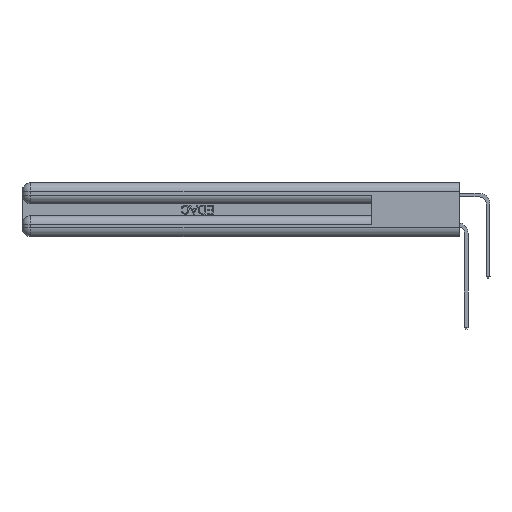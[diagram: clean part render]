
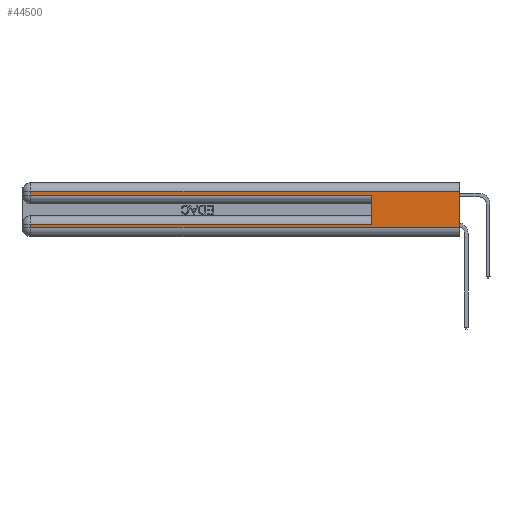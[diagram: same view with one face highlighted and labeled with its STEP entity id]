
A CAD part, left-side view. The second image highlights one B-rep face of the part: STEP entity #44500.
In plain terms, the highlighted planar face has unit normal (-1, 0, 0).
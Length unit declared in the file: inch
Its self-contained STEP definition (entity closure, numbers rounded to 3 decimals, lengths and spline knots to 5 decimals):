
#32 = LINE ( 'NONE', #15522, #5811 ) ;
#639 = VECTOR ( 'NONE', #29150, 39.37008 ) ;
#672 = VECTOR ( 'NONE', #7883, 39.37008 ) ;
#2820 = EDGE_CURVE ( 'NONE', #15118, #32113, #42687, .T. ) ;
#3298 = VERTEX_POINT ( 'NONE', #42536 ) ;
#4163 = VERTEX_POINT ( 'NONE', #35458 ) ;
#4342 = CARTESIAN_POINT ( 'NONE',  ( 0., 0., 0.31 ) ) ;
#5330 = DIRECTION ( 'NONE',  ( 0., 0., -1. ) ) ;
#5811 = VECTOR ( 'NONE', #40610, 39.37008 ) ;
#5870 = CARTESIAN_POINT ( 'NONE',  ( 0., 0., 0.06 ) ) ;
#6993 = AXIS2_PLACEMENT_3D ( 'NONE', #20928, #46917, #7192 ) ;
#7192 = DIRECTION ( 'NONE',  ( 0., 0., -1. ) ) ;
#7569 = LINE ( 'NONE', #17397, #22029 ) ;
#7586 = DIRECTION ( 'NONE',  ( 0., 0., -1. ) ) ;
#7883 = DIRECTION ( 'NONE',  ( 0., 1., 0. ) ) ;
#8576 = ORIENTED_EDGE ( 'NONE', *, *, #2820, .T. ) ;
#9760 = ORIENTED_EDGE ( 'NONE', *, *, #25364, .T. ) ;
#10143 = LINE ( 'NONE', #27771, #14815 ) ;
#13827 = DIRECTION ( 'NONE',  ( 0., 1., 0. ) ) ;
#13920 = LINE ( 'NONE', #4342, #672 ) ;
#14439 = VECTOR ( 'NONE', #7586, 39.37008 ) ;
#14815 = VECTOR ( 'NONE', #5330, 39.37008 ) ;
#15118 = VERTEX_POINT ( 'NONE', #22848 ) ;
#15131 = VERTEX_POINT ( 'NONE', #5870 ) ;
#15522 = CARTESIAN_POINT ( 'NONE',  ( 0., 2.94, 0.37 ) ) ;
#17222 = EDGE_CURVE ( 'NONE', #34478, #18500, #39340, .T. ) ;
#17397 = CARTESIAN_POINT ( 'NONE',  ( 0., 0., 0.085 ) ) ;
#18054 = EDGE_CURVE ( 'NONE', #20332, #4163, #32, .T. ) ;
#18500 = VERTEX_POINT ( 'NONE', #32402 ) ;
#20332 = VERTEX_POINT ( 'NONE', #34248 ) ;
#20928 = CARTESIAN_POINT ( 'NONE',  ( 0., 0., 0.37 ) ) ;
#21116 = EDGE_CURVE ( 'NONE', #3298, #15131, #10143, .T. ) ;
#21173 = ORIENTED_EDGE ( 'NONE', *, *, #21116, .F. ) ;
#21985 = CARTESIAN_POINT ( 'NONE',  ( 0., 0.6, 0.085 ) ) ;
#22029 = VECTOR ( 'NONE', #13827, 39.37008 ) ;
#22497 = EDGE_LOOP ( 'NONE', ( #21173, #37369, #8576, #9760, #22871, #39347, #37318, #46842 ) ) ;
#22683 = CARTESIAN_POINT ( 'NONE',  ( 0., 2.94, 0.37 ) ) ;
#22848 = CARTESIAN_POINT ( 'NONE',  ( 0., 2.94, 0.31 ) ) ;
#22871 = ORIENTED_EDGE ( 'NONE', *, *, #17222, .F. ) ;
#23947 = EDGE_CURVE ( 'NONE', #34478, #20332, #7569, .T. ) ;
#24166 = FACE_OUTER_BOUND ( 'NONE', #22497, .T. ) ;
#25364 = EDGE_CURVE ( 'NONE', #32113, #18500, #36343, .T. ) ;
#27719 = CARTESIAN_POINT ( 'NONE',  ( 0., 0., 0.06 ) ) ;
#27771 = CARTESIAN_POINT ( 'NONE',  ( 0., 0., 0.37 ) ) ;
#29150 = DIRECTION ( 'NONE',  ( 0., -1., 0. ) ) ;
#31584 = CARTESIAN_POINT ( 'NONE',  ( 0., 0.6, 0.145 ) ) ;
#32113 = VERTEX_POINT ( 'NONE', #34582 ) ;
#32402 = CARTESIAN_POINT ( 'NONE',  ( 0., 0.6, 0.285 ) ) ;
#34248 = CARTESIAN_POINT ( 'NONE',  ( 0., 2.94, 0.085 ) ) ;
#34478 = VERTEX_POINT ( 'NONE', #21985 ) ;
#34582 = CARTESIAN_POINT ( 'NONE',  ( 0., 2.94, 0.285 ) ) ;
#35062 = VECTOR ( 'NONE', #42788, 39.37008 ) ;
#35458 = CARTESIAN_POINT ( 'NONE',  ( 0., 2.94, 0.06 ) ) ;
#36342 = CARTESIAN_POINT ( 'NONE',  ( 0., 0., 0.285 ) ) ;
#36343 = LINE ( 'NONE', #36342, #639 ) ;
#37318 = ORIENTED_EDGE ( 'NONE', *, *, #18054, .T. ) ;
#37369 = ORIENTED_EDGE ( 'NONE', *, *, #42899, .T. ) ;
#37616 = VECTOR ( 'NONE', #46282, 39.37008 ) ;
#38562 = LINE ( 'NONE', #27719, #35062 ) ;
#39340 = LINE ( 'NONE', #31584, #37616 ) ;
#39347 = ORIENTED_EDGE ( 'NONE', *, *, #23947, .T. ) ;
#40610 = DIRECTION ( 'NONE',  ( 0., 0., -1. ) ) ;
#42536 = CARTESIAN_POINT ( 'NONE',  ( 0., 0., 0.31 ) ) ;
#42687 = LINE ( 'NONE', #22683, #14439 ) ;
#42788 = DIRECTION ( 'NONE',  ( 0., -1., 0. ) ) ;
#42819 = PLANE ( 'NONE',  #6993 ) ;
#42899 = EDGE_CURVE ( 'NONE', #3298, #15118, #13920, .T. ) ;
#44500 = ADVANCED_FACE ( 'NONE', ( #24166 ), #42819, .F. ) ;
#44952 = EDGE_CURVE ( 'NONE', #4163, #15131, #38562, .T. ) ;
#46282 = DIRECTION ( 'NONE',  ( 0., 0., 1. ) ) ;
#46842 = ORIENTED_EDGE ( 'NONE', *, *, #44952, .T. ) ;
#46917 = DIRECTION ( 'NONE',  ( 1., 0., 0. ) ) ;
